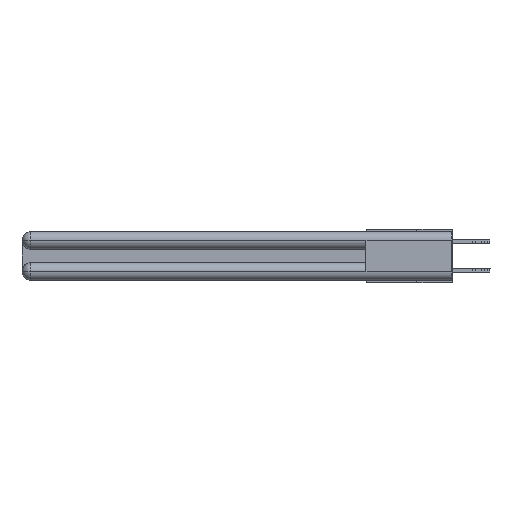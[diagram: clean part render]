
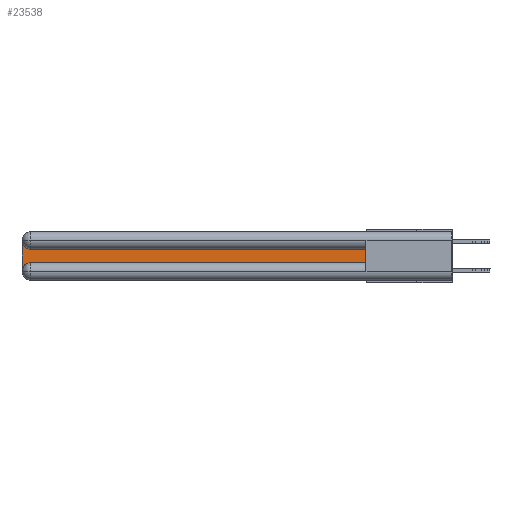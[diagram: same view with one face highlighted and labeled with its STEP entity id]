
A CAD part, left-side view. The second image highlights one B-rep face of the part: STEP entity #23538.
In plain terms, the highlighted planar face has unit normal (-1, 0, 0).
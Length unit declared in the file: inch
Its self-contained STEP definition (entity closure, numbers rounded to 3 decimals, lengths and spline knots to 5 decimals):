
#572 = EDGE_CURVE ( 'NONE', #20877, #23555, #15170, .T. ) ;
#2049 = DIRECTION ( 'NONE',  ( 0., 0., -1. ) ) ;
#2664 = CARTESIAN_POINT ( 'NONE',  ( 0.075, 0.6, -0.1225 ) ) ;
#3151 = AXIS2_PLACEMENT_3D ( 'NONE', #14041, #27425, #13842 ) ;
#4104 = VECTOR ( 'NONE', #12193, 39.37008 ) ;
#4259 = DIRECTION ( 'NONE',  ( 1., 0., 0. ) ) ;
#4534 = VECTOR ( 'NONE', #26689, 39.37008 ) ;
#4610 = DIRECTION ( 'NONE',  ( 0., 0., -1. ) ) ;
#4779 = FACE_OUTER_BOUND ( 'NONE', #23753, .T. ) ;
#5612 = VERTEX_POINT ( 'NONE', #2664 ) ;
#5801 = VERTEX_POINT ( 'NONE', #8939 ) ;
#6036 = ORIENTED_EDGE ( 'NONE', *, *, #12380, .T. ) ;
#6093 = CARTESIAN_POINT ( 'NONE',  ( 0.075, 0.6, -0.1225 ) ) ;
#6273 = ORIENTED_EDGE ( 'NONE', *, *, #26444, .T. ) ;
#6814 = CARTESIAN_POINT ( 'NONE',  ( 0.075, 0.6, -0.2175 ) ) ;
#7639 = CARTESIAN_POINT ( 'NONE',  ( 0.075, 0.6, -0.2175 ) ) ;
#7729 = CARTESIAN_POINT ( 'NONE',  ( 0.075, 0.6, -0.2175 ) ) ;
#8777 = PLANE ( 'NONE',  #10496 ) ;
#8939 = CARTESIAN_POINT ( 'NONE',  ( 0.075, 2.94, -0.2175 ) ) ;
#9742 = CIRCLE ( 'NONE', #19930, 0.06 ) ;
#10496 = AXIS2_PLACEMENT_3D ( 'NONE', #20219, #24619, #4610 ) ;
#11751 = CARTESIAN_POINT ( 'NONE',  ( 0.075, 2.94, -0.1225 ) ) ;
#11923 = LINE ( 'NONE', #7729, #17902 ) ;
#12193 = DIRECTION ( 'NONE',  ( 0., -1., 0. ) ) ;
#12380 = EDGE_CURVE ( 'NONE', #14713, #5612, #11923, .T. ) ;
#12627 = ORIENTED_EDGE ( 'NONE', *, *, #22785, .T. ) ;
#13252 = CARTESIAN_POINT ( 'NONE',  ( 0.075, 2.94, -0.2775 ) ) ;
#13489 = ORIENTED_EDGE ( 'NONE', *, *, #572, .T. ) ;
#13842 = DIRECTION ( 'NONE',  ( 0., 0., -1. ) ) ;
#14041 = CARTESIAN_POINT ( 'NONE',  ( 0.075, 2.94, -0.0625 ) ) ;
#14340 = VERTEX_POINT ( 'NONE', #14353 ) ;
#14353 = CARTESIAN_POINT ( 'NONE',  ( 0.075, 3., -0.2775 ) ) ;
#14713 = VERTEX_POINT ( 'NONE', #6814 ) ;
#14727 = DIRECTION ( 'NONE',  ( 0., 0., 1. ) ) ;
#15143 = LINE ( 'NONE', #6093, #4534 ) ;
#15170 = CIRCLE ( 'NONE', #3151, 0.06 ) ;
#15511 = DIRECTION ( 'NONE',  ( 0., 0., -1. ) ) ;
#17902 = VECTOR ( 'NONE', #14727, 39.37008 ) ;
#19930 = AXIS2_PLACEMENT_3D ( 'NONE', #13252, #4259, #15511 ) ;
#20219 = CARTESIAN_POINT ( 'NONE',  ( 0.075, 3., -0.1225 ) ) ;
#20508 = CARTESIAN_POINT ( 'NONE',  ( 0.075, 3., -0.0625 ) ) ;
#20877 = VERTEX_POINT ( 'NONE', #11751 ) ;
#21872 = CARTESIAN_POINT ( 'NONE',  ( 0.075, 3., -0.2175 ) ) ;
#22556 = ORIENTED_EDGE ( 'NONE', *, *, #27732, .T. ) ;
#22785 = EDGE_CURVE ( 'NONE', #5801, #14713, #28923, .T. ) ;
#23538 = ADVANCED_FACE ( 'NONE', ( #4779 ), #8777, .F. ) ;
#23555 = VERTEX_POINT ( 'NONE', #20508 ) ;
#23753 = EDGE_LOOP ( 'NONE', ( #22556, #13489, #6273, #26679, #12627, #6036 ) ) ;
#24260 = EDGE_CURVE ( 'NONE', #14340, #5801, #9742, .T. ) ;
#24441 = VECTOR ( 'NONE', #2049, 39.37008 ) ;
#24619 = DIRECTION ( 'NONE',  ( 1., 0., 0. ) ) ;
#24798 = LINE ( 'NONE', #21872, #24441 ) ;
#26444 = EDGE_CURVE ( 'NONE', #23555, #14340, #24798, .T. ) ;
#26679 = ORIENTED_EDGE ( 'NONE', *, *, #24260, .T. ) ;
#26689 = DIRECTION ( 'NONE',  ( 0., 1., 0. ) ) ;
#27425 = DIRECTION ( 'NONE',  ( 1., 0., 0. ) ) ;
#27732 = EDGE_CURVE ( 'NONE', #5612, #20877, #15143, .T. ) ;
#28923 = LINE ( 'NONE', #7639, #4104 ) ;
